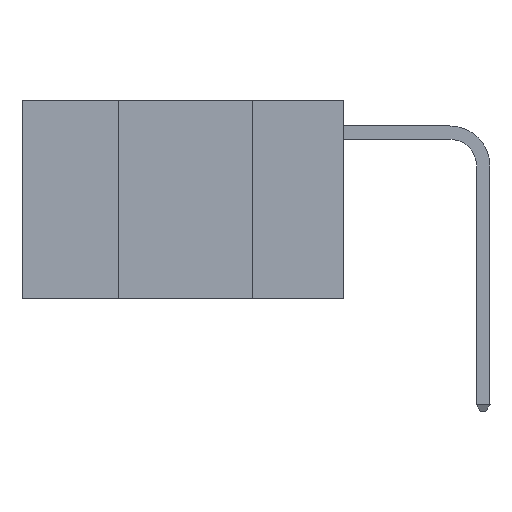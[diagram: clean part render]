
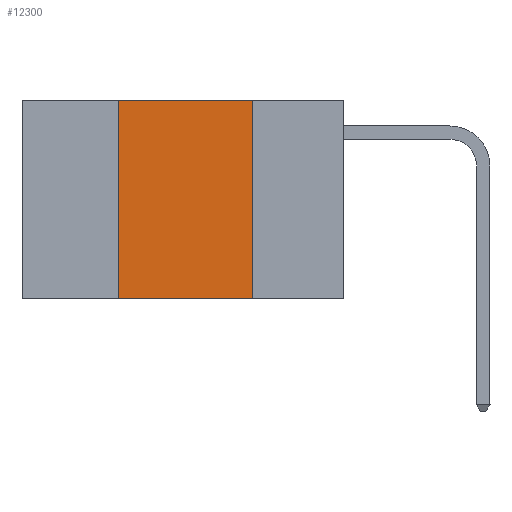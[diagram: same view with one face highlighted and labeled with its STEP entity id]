
A CAD part, left-side view. The second image highlights one B-rep face of the part: STEP entity #12300.
In plain terms, the highlighted planar face has unit normal (-1, 0, 0).
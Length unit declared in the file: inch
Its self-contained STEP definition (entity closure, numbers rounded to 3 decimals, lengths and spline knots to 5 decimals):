
#417 = LINE ( 'NONE', #8271, #7125 ) ;
#814 = VECTOR ( 'NONE', #10471, 39.37008 ) ;
#1327 = DIRECTION ( 'NONE',  ( 1., 0., 0. ) ) ;
#1665 = AXIS2_PLACEMENT_3D ( 'NONE', #9833, #1327, #11217 ) ;
#2007 = CARTESIAN_POINT ( 'NONE',  ( 0., 0.17, 0. ) ) ;
#2991 = CARTESIAN_POINT ( 'NONE',  ( 0., 0.17, -0.37 ) ) ;
#3190 = CARTESIAN_POINT ( 'NONE',  ( 0., 0.42, 0. ) ) ;
#4073 = FACE_OUTER_BOUND ( 'NONE', #17705, .T. ) ;
#4997 = LINE ( 'NONE', #16221, #5445 ) ;
#5281 = EDGE_CURVE ( 'NONE', #8279, #9447, #4997, .T. ) ;
#5445 = VECTOR ( 'NONE', #8043, 39.37008 ) ;
#7089 = ORIENTED_EDGE ( 'NONE', *, *, #7597, .F. ) ;
#7125 = VECTOR ( 'NONE', #15102, 39.37008 ) ;
#7133 = ORIENTED_EDGE ( 'NONE', *, *, #11201, .F. ) ;
#7148 = ORIENTED_EDGE ( 'NONE', *, *, #13414, .F. ) ;
#7250 = ORIENTED_EDGE ( 'NONE', *, *, #5281, .T. ) ;
#7597 = EDGE_CURVE ( 'NONE', #17126, #9447, #8420, .T. ) ;
#8043 = DIRECTION ( 'NONE',  ( 0., -1., 0. ) ) ;
#8115 = VECTOR ( 'NONE', #13088, 39.37008 ) ;
#8271 = CARTESIAN_POINT ( 'NONE',  ( 0., 0.42, 0. ) ) ;
#8279 = VERTEX_POINT ( 'NONE', #8869 ) ;
#8420 = LINE ( 'NONE', #2007, #814 ) ;
#8869 = CARTESIAN_POINT ( 'NONE',  ( 0., 0.42, -0.37 ) ) ;
#9447 = VERTEX_POINT ( 'NONE', #2991 ) ;
#9833 = CARTESIAN_POINT ( 'NONE',  ( 0., 0.6, 0. ) ) ;
#10471 = DIRECTION ( 'NONE',  ( 0., 0., -1. ) ) ;
#11201 = EDGE_CURVE ( 'NONE', #13132, #17126, #15392, .T. ) ;
#11217 = DIRECTION ( 'NONE',  ( 0., 0., -1. ) ) ;
#11685 = CARTESIAN_POINT ( 'NONE',  ( 0., 0.6, 0. ) ) ;
#12300 = ADVANCED_FACE ( 'NONE', ( #4073 ), #17861, .F. ) ;
#12454 = CARTESIAN_POINT ( 'NONE',  ( 0., 0.17, 0. ) ) ;
#13088 = DIRECTION ( 'NONE',  ( 0., -1., 0. ) ) ;
#13132 = VERTEX_POINT ( 'NONE', #3190 ) ;
#13414 = EDGE_CURVE ( 'NONE', #8279, #13132, #417, .T. ) ;
#15102 = DIRECTION ( 'NONE',  ( 0., 0., 1. ) ) ;
#15392 = LINE ( 'NONE', #11685, #8115 ) ;
#16221 = CARTESIAN_POINT ( 'NONE',  ( 0., 0.6, -0.37 ) ) ;
#17126 = VERTEX_POINT ( 'NONE', #12454 ) ;
#17705 = EDGE_LOOP ( 'NONE', ( #7089, #7133, #7148, #7250 ) ) ;
#17861 = PLANE ( 'NONE',  #1665 ) ;
